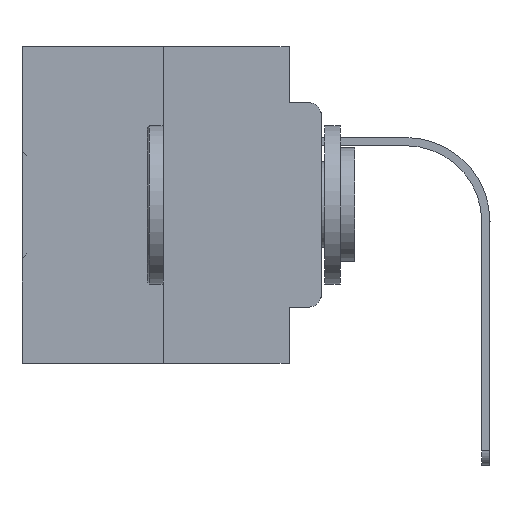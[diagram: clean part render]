
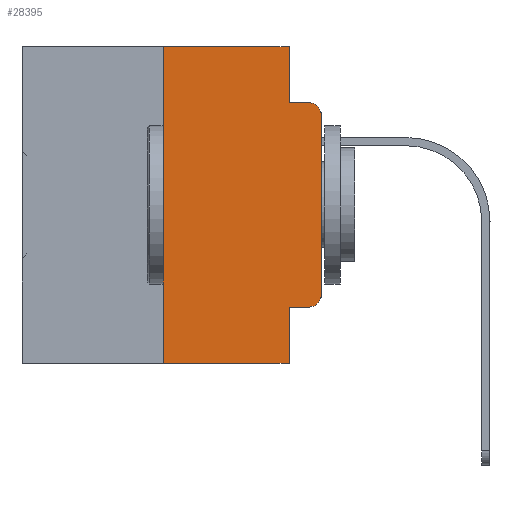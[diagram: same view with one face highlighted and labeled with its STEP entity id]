
A CAD part, left-side view. The second image highlights one B-rep face of the part: STEP entity #28395.
In plain terms, the highlighted planar face has unit normal (-1, 0, 0).
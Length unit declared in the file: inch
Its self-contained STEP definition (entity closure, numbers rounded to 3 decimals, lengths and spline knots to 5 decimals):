
#422 = CARTESIAN_POINT ( 'NONE',  ( 0., 0., -0.3915 ) ) ;
#769 = ORIENTED_EDGE ( 'NONE', *, *, #25200, .T. ) ;
#1169 = VECTOR ( 'NONE', #33615, 39.37008 ) ;
#1933 = ORIENTED_EDGE ( 'NONE', *, *, #13085, .F. ) ;
#2738 = LINE ( 'NONE', #13551, #28321 ) ;
#2787 = ORIENTED_EDGE ( 'NONE', *, *, #8467, .F. ) ;
#3984 = VERTEX_POINT ( 'NONE', #19380 ) ;
#4000 = CARTESIAN_POINT ( 'NONE',  ( 0., 0.051, -0.4115 ) ) ;
#4355 = VERTEX_POINT ( 'NONE', #34067 ) ;
#4507 = LINE ( 'NONE', #29280, #15576 ) ;
#5486 = VERTEX_POINT ( 'NONE', #33434 ) ;
#6632 = DIRECTION ( 'NONE',  ( -1., 0., 0. ) ) ;
#6842 = VERTEX_POINT ( 'NONE', #29005 ) ;
#6845 = LINE ( 'NONE', #20117, #34722 ) ;
#6891 = CARTESIAN_POINT ( 'NONE',  ( 0., 0.25, 0. ) ) ;
#7346 = CARTESIAN_POINT ( 'NONE',  ( 0., 0.02, -0.1085 ) ) ;
#7936 = VERTEX_POINT ( 'NONE', #26646 ) ;
#8467 = EDGE_CURVE ( 'NONE', #27349, #30285, #21278, .T. ) ;
#8673 = AXIS2_PLACEMENT_3D ( 'NONE', #11434, #21860, #22394 ) ;
#10266 = CARTESIAN_POINT ( 'NONE',  ( 0., 0.473, -0.5 ) ) ;
#10460 = CARTESIAN_POINT ( 'NONE',  ( 0., 0.02, -0.0885 ) ) ;
#11285 = CARTESIAN_POINT ( 'NONE',  ( 0., 0., -0.1085 ) ) ;
#11370 = VECTOR ( 'NONE', #11627, 39.37008 ) ;
#11434 = CARTESIAN_POINT ( 'NONE',  ( 0., 0.02, -0.3915 ) ) ;
#11627 = DIRECTION ( 'NONE',  ( 0., -1., 0. ) ) ;
#11702 = CARTESIAN_POINT ( 'NONE',  ( 0., 0.473, 0. ) ) ;
#12149 = LINE ( 'NONE', #4000, #11370 ) ;
#12506 = EDGE_CURVE ( 'NONE', #6842, #4355, #6845, .T. ) ;
#13008 = DIRECTION ( 'NONE',  ( 0., 0., -1. ) ) ;
#13085 = EDGE_CURVE ( 'NONE', #4355, #7936, #4507, .T. ) ;
#13199 = CIRCLE ( 'NONE', #25605, 0.02 ) ;
#13551 = CARTESIAN_POINT ( 'NONE',  ( 0., 0., 0. ) ) ;
#15241 = PLANE ( 'NONE',  #30180 ) ;
#15576 = VECTOR ( 'NONE', #13008, 39.37008 ) ;
#16501 = DIRECTION ( 'NONE',  ( 0., 0., -1. ) ) ;
#16734 = CARTESIAN_POINT ( 'NONE',  ( 0., 0.051, -0.4115 ) ) ;
#17240 = VECTOR ( 'NONE', #16501, 39.37008 ) ;
#17802 = DIRECTION ( 'NONE',  ( 0., -1., 0. ) ) ;
#18450 = EDGE_CURVE ( 'NONE', #3984, #30285, #26883, .T. ) ;
#18484 = DIRECTION ( 'NONE',  ( 0., 0., 1. ) ) ;
#18708 = CARTESIAN_POINT ( 'NONE',  ( 0., 0.051, -0.5 ) ) ;
#18731 = DIRECTION ( 'NONE',  ( 0., -1., 0. ) ) ;
#18745 = ORIENTED_EDGE ( 'NONE', *, *, #27329, .T. ) ;
#19380 = CARTESIAN_POINT ( 'NONE',  ( 0., 0.25, -0.5 ) ) ;
#19547 = LINE ( 'NONE', #29833, #24950 ) ;
#20117 = CARTESIAN_POINT ( 'NONE',  ( 0., 0.473, 0. ) ) ;
#20841 = VERTEX_POINT ( 'NONE', #11285 ) ;
#21147 = ORIENTED_EDGE ( 'NONE', *, *, #18450, .T. ) ;
#21278 = LINE ( 'NONE', #32078, #17240 ) ;
#21860 = DIRECTION ( 'NONE',  ( -1., 0., 0. ) ) ;
#21879 = EDGE_CURVE ( 'NONE', #3984, #6842, #28657, .T. ) ;
#22394 = DIRECTION ( 'NONE',  ( 0., 0., -1. ) ) ;
#22490 = DIRECTION ( 'NONE',  ( 0., 0., -1. ) ) ;
#22574 = EDGE_CURVE ( 'NONE', #7936, #25740, #19547, .T. ) ;
#23770 = EDGE_CURVE ( 'NONE', #23921, #20841, #2738, .T. ) ;
#23836 = ORIENTED_EDGE ( 'NONE', *, *, #22574, .F. ) ;
#23921 = VERTEX_POINT ( 'NONE', #422 ) ;
#24048 = ORIENTED_EDGE ( 'NONE', *, *, #23770, .T. ) ;
#24950 = VECTOR ( 'NONE', #27357, 39.37008 ) ;
#25200 = EDGE_CURVE ( 'NONE', #27349, #5486, #12149, .T. ) ;
#25605 = AXIS2_PLACEMENT_3D ( 'NONE', #7346, #6632, #28955 ) ;
#25663 = DIRECTION ( 'NONE',  ( 1., 0., 0. ) ) ;
#25740 = VERTEX_POINT ( 'NONE', #10460 ) ;
#25751 = ORIENTED_EDGE ( 'NONE', *, *, #12506, .F. ) ;
#26402 = ORIENTED_EDGE ( 'NONE', *, *, #27487, .T. ) ;
#26646 = CARTESIAN_POINT ( 'NONE',  ( 0., 0.051, -0.0885 ) ) ;
#26883 = LINE ( 'NONE', #10266, #27088 ) ;
#27061 = ORIENTED_EDGE ( 'NONE', *, *, #21879, .F. ) ;
#27088 = VECTOR ( 'NONE', #18731, 39.37008 ) ;
#27329 = EDGE_CURVE ( 'NONE', #5486, #23921, #30724, .T. ) ;
#27349 = VERTEX_POINT ( 'NONE', #16734 ) ;
#27357 = DIRECTION ( 'NONE',  ( 0., -1., 0. ) ) ;
#27487 = EDGE_CURVE ( 'NONE', #20841, #25740, #13199, .T. ) ;
#28321 = VECTOR ( 'NONE', #18484, 39.37008 ) ;
#28395 = ADVANCED_FACE ( 'NONE', ( #28675 ), #15241, .F. ) ;
#28657 = LINE ( 'NONE', #6891, #1169 ) ;
#28675 = FACE_OUTER_BOUND ( 'NONE', #31458, .T. ) ;
#28955 = DIRECTION ( 'NONE',  ( 0., 0., -1. ) ) ;
#29005 = CARTESIAN_POINT ( 'NONE',  ( 0., 0.25, 0. ) ) ;
#29280 = CARTESIAN_POINT ( 'NONE',  ( 0., 0.051, 0. ) ) ;
#29833 = CARTESIAN_POINT ( 'NONE',  ( 0., 0.051, -0.0885 ) ) ;
#30180 = AXIS2_PLACEMENT_3D ( 'NONE', #11702, #25663, #22490 ) ;
#30285 = VERTEX_POINT ( 'NONE', #18708 ) ;
#30724 = CIRCLE ( 'NONE', #8673, 0.02 ) ;
#31458 = EDGE_LOOP ( 'NONE', ( #24048, #26402, #23836, #1933, #25751, #27061, #21147, #2787, #769, #18745 ) ) ;
#32078 = CARTESIAN_POINT ( 'NONE',  ( 0., 0.051, 0. ) ) ;
#33434 = CARTESIAN_POINT ( 'NONE',  ( 0., 0.02, -0.4115 ) ) ;
#33615 = DIRECTION ( 'NONE',  ( 0., 0., 1. ) ) ;
#34067 = CARTESIAN_POINT ( 'NONE',  ( 0., 0.051, 0. ) ) ;
#34722 = VECTOR ( 'NONE', #17802, 39.37008 ) ;
